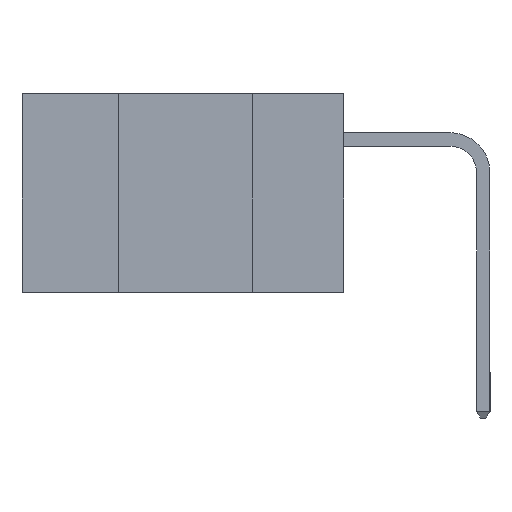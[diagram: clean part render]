
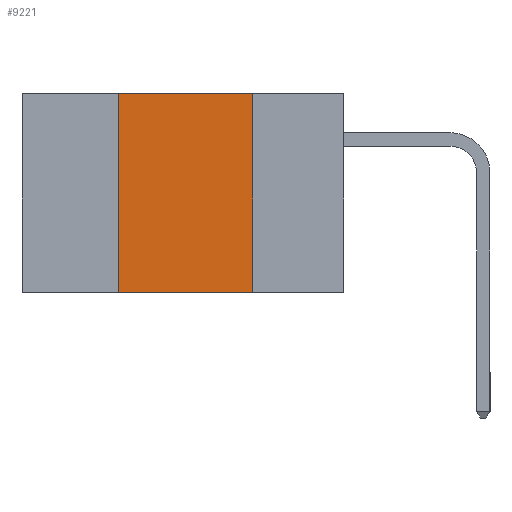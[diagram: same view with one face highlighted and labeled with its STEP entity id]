
A CAD part, left-side view. The second image highlights one B-rep face of the part: STEP entity #9221.
In plain terms, the highlighted planar face has unit normal (-1, 0, 0).
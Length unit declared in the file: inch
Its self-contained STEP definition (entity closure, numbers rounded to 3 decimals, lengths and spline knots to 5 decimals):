
#28 = DIRECTION ( 'NONE',  ( 1., 0., 0. ) ) ;
#1980 = EDGE_CURVE ( 'NONE', #5525, #6284, #5126, .T. ) ;
#2034 = ORIENTED_EDGE ( 'NONE', *, *, #7982, .F. ) ;
#2712 = ORIENTED_EDGE ( 'NONE', *, *, #7970, .T. ) ;
#3501 = CARTESIAN_POINT ( 'NONE',  ( 0., 0.6, -0.37 ) ) ;
#3502 = VERTEX_POINT ( 'NONE', #3841 ) ;
#3580 = VECTOR ( 'NONE', #10019, 39.37008 ) ;
#3841 = CARTESIAN_POINT ( 'NONE',  ( 0., 0.17, -0.37 ) ) ;
#3950 = VECTOR ( 'NONE', #4854, 39.37008 ) ;
#4087 = DIRECTION ( 'NONE',  ( 0., 0., -1. ) ) ;
#4094 = ORIENTED_EDGE ( 'NONE', *, *, #1980, .F. ) ;
#4854 = DIRECTION ( 'NONE',  ( 0., -1., 0. ) ) ;
#4924 = EDGE_CURVE ( 'NONE', #6284, #5421, #8054, .T. ) ;
#4938 = CARTESIAN_POINT ( 'NONE',  ( 0., 0.6, 0. ) ) ;
#4996 = CARTESIAN_POINT ( 'NONE',  ( 0., 0.6, 0. ) ) ;
#5126 = LINE ( 'NONE', #5192, #3580 ) ;
#5192 = CARTESIAN_POINT ( 'NONE',  ( 0., 0.42, 0. ) ) ;
#5421 = VERTEX_POINT ( 'NONE', #6885 ) ;
#5525 = VERTEX_POINT ( 'NONE', #6953 ) ;
#5595 = DIRECTION ( 'NONE',  ( 0., 0., -1. ) ) ;
#5936 = PLANE ( 'NONE',  #11887 ) ;
#6027 = VECTOR ( 'NONE', #5595, 39.37008 ) ;
#6284 = VERTEX_POINT ( 'NONE', #6318 ) ;
#6318 = CARTESIAN_POINT ( 'NONE',  ( 0., 0.42, 0. ) ) ;
#6885 = CARTESIAN_POINT ( 'NONE',  ( 0., 0.17, 0. ) ) ;
#6953 = CARTESIAN_POINT ( 'NONE',  ( 0., 0.42, -0.37 ) ) ;
#6977 = VECTOR ( 'NONE', #8576, 39.37008 ) ;
#7970 = EDGE_CURVE ( 'NONE', #5525, #3502, #9938, .T. ) ;
#7982 = EDGE_CURVE ( 'NONE', #5421, #3502, #11657, .T. ) ;
#8054 = LINE ( 'NONE', #4938, #3950 ) ;
#8576 = DIRECTION ( 'NONE',  ( 0., -1., 0. ) ) ;
#8766 = ORIENTED_EDGE ( 'NONE', *, *, #4924, .F. ) ;
#8959 = FACE_OUTER_BOUND ( 'NONE', #11143, .T. ) ;
#9221 = ADVANCED_FACE ( 'NONE', ( #8959 ), #5936, .F. ) ;
#9938 = LINE ( 'NONE', #3501, #6977 ) ;
#10019 = DIRECTION ( 'NONE',  ( 0., 0., 1. ) ) ;
#11143 = EDGE_LOOP ( 'NONE', ( #2034, #8766, #4094, #2712 ) ) ;
#11591 = CARTESIAN_POINT ( 'NONE',  ( 0., 0.17, 0. ) ) ;
#11657 = LINE ( 'NONE', #11591, #6027 ) ;
#11887 = AXIS2_PLACEMENT_3D ( 'NONE', #4996, #28, #4087 ) ;
